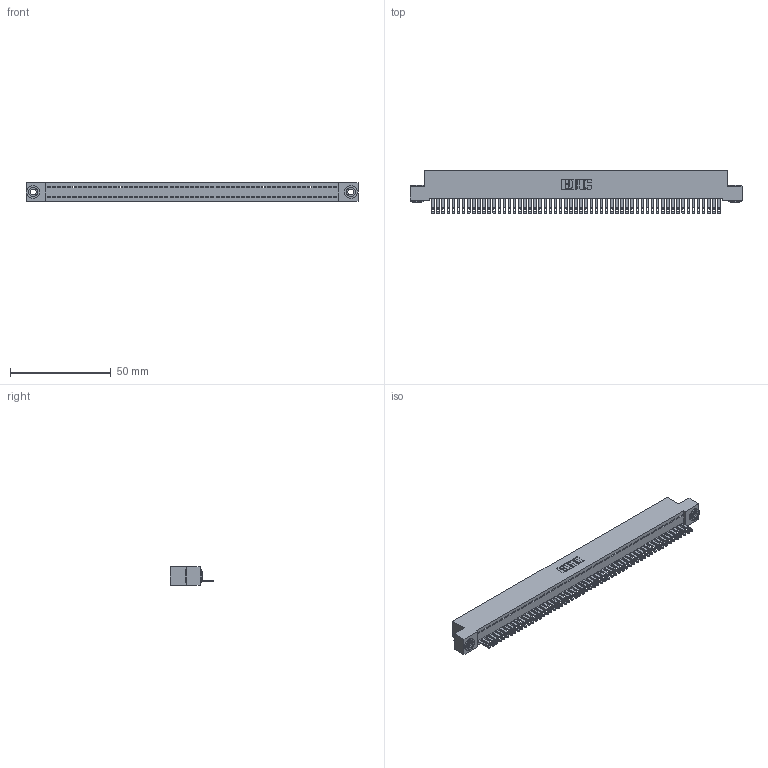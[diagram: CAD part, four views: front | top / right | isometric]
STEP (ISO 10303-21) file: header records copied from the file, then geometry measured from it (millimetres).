
FILE_DESCRIPTION (( 'STEP AP203' ), '1' );
FILE_NAME ('342-057-500-103.STEP', '2018-08-13T04:15:53', ( '' ), ( '' ), 'SwSTEP 2.0', 'SolidWorks 2016', '' );
FILE_SCHEMA (( 'CONFIG_CONTROL_DESIGN' ));
Length unit declared in the file: inch
Products named in the file (4): 342 Part_.156 TH; 345-292-001_345-293-100; 342-250-002_345-250-002-102; 342-057-500-103
Assembly tree (60 placements, depth 2):
  342-057-500-103
    342 Part_.156 TH
    345-292-001_345-293-100  x57
    342-250-002_345-250-002-102  x2
Bounding box: 165.1 x 21.85 x 9.4 mm (x, y, z)
Volume: 14589.3 mm3; surface area: 22042.2 mm2
Topology: 60 solids, 60 shells, 3226 faces, 9951 edges, 6630 vertices
Faces by surface type: plane 2128, cylinder 1090, cone 8
Entity records: 33354 total; most frequent: CARTESIAN_POINT 5728, ORIENTED_EDGE 5714, DIRECTION 4837, EDGE_CURVE 2857, VECTOR 2701, LINE 2701, VERTEX_POINT 1902, AXIS2_PLACEMENT_3D 1068
